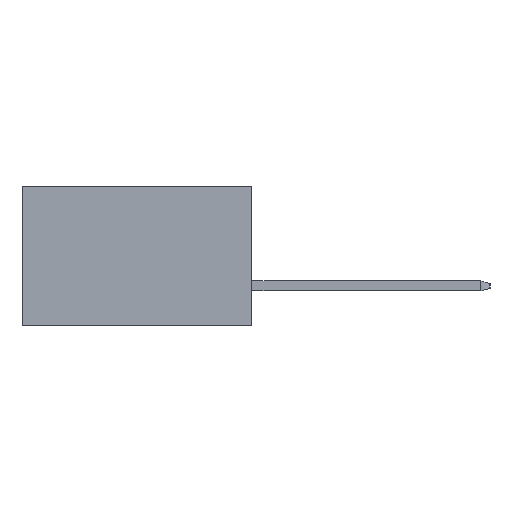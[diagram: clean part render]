
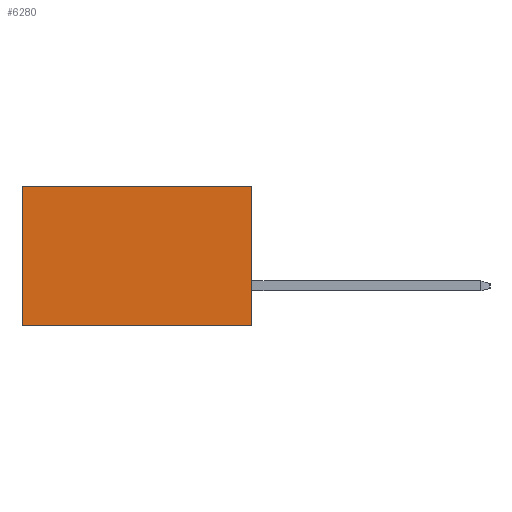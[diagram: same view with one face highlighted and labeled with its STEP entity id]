
A CAD part, left-side view. The second image highlights one B-rep face of the part: STEP entity #6280.
In plain terms, the highlighted planar face has unit normal (-1, 0, 0).
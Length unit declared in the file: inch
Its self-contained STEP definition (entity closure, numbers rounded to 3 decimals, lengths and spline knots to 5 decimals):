
#103 = AXIS2_PLACEMENT_3D ( 'NONE', #6134, #9323, #2101 ) ;
#768 = ORIENTED_EDGE ( 'NONE', *, *, #8741, .F. ) ;
#1067 = DIRECTION ( 'NONE',  ( 0., 1., 0. ) ) ;
#1309 = EDGE_CURVE ( 'NONE', #7422, #1855, #4258, .T. ) ;
#1829 = LINE ( 'NONE', #1872, #4483 ) ;
#1855 = VERTEX_POINT ( 'NONE', #2304 ) ;
#1872 = CARTESIAN_POINT ( 'NONE',  ( 0.3205, 0.72, -0.437 ) ) ;
#2050 = PLANE ( 'NONE',  #103 ) ;
#2101 = DIRECTION ( 'NONE',  ( 0., 0., -1. ) ) ;
#2162 = ORIENTED_EDGE ( 'NONE', *, *, #7041, .T. ) ;
#2304 = CARTESIAN_POINT ( 'NONE',  ( 0.3205, 0.72, 0. ) ) ;
#2458 = CARTESIAN_POINT ( 'NONE',  ( 0.3205, 0., 0. ) ) ;
#2669 = DIRECTION ( 'NONE',  ( 0., 0., -1. ) ) ;
#3473 = CARTESIAN_POINT ( 'NONE',  ( 0.3205, 0.72, -0.437 ) ) ;
#3749 = FACE_OUTER_BOUND ( 'NONE', #8876, .T. ) ;
#4103 = LINE ( 'NONE', #7506, #8372 ) ;
#4258 = LINE ( 'NONE', #7366, #6295 ) ;
#4483 = VECTOR ( 'NONE', #5948, 39.37008 ) ;
#4635 = CARTESIAN_POINT ( 'NONE',  ( 0.3205, 0., -0.437 ) ) ;
#4843 = LINE ( 'NONE', #6491, #9680 ) ;
#5049 = DIRECTION ( 'NONE',  ( 0., 1., 0. ) ) ;
#5707 = EDGE_CURVE ( 'NONE', #6292, #6922, #4843, .T. ) ;
#5948 = DIRECTION ( 'NONE',  ( 0., 0., -1. ) ) ;
#5989 = ORIENTED_EDGE ( 'NONE', *, *, #5707, .F. ) ;
#6134 = CARTESIAN_POINT ( 'NONE',  ( 0.3205, 0., -0.437 ) ) ;
#6280 = ADVANCED_FACE ( 'NONE', ( #3749 ), #2050, .F. ) ;
#6292 = VERTEX_POINT ( 'NONE', #4635 ) ;
#6295 = VECTOR ( 'NONE', #1067, 39.37008 ) ;
#6491 = CARTESIAN_POINT ( 'NONE',  ( 0.3205, 0., -0.437 ) ) ;
#6913 = ORIENTED_EDGE ( 'NONE', *, *, #1309, .T. ) ;
#6922 = VERTEX_POINT ( 'NONE', #3473 ) ;
#7041 = EDGE_CURVE ( 'NONE', #1855, #6922, #1829, .T. ) ;
#7366 = CARTESIAN_POINT ( 'NONE',  ( 0.3205, 0., 0. ) ) ;
#7422 = VERTEX_POINT ( 'NONE', #2458 ) ;
#7506 = CARTESIAN_POINT ( 'NONE',  ( 0.3205, 0., -0.437 ) ) ;
#8372 = VECTOR ( 'NONE', #2669, 39.37008 ) ;
#8741 = EDGE_CURVE ( 'NONE', #7422, #6292, #4103, .T. ) ;
#8876 = EDGE_LOOP ( 'NONE', ( #2162, #5989, #768, #6913 ) ) ;
#9323 = DIRECTION ( 'NONE',  ( 1., 0., 0. ) ) ;
#9680 = VECTOR ( 'NONE', #5049, 39.37008 ) ;
